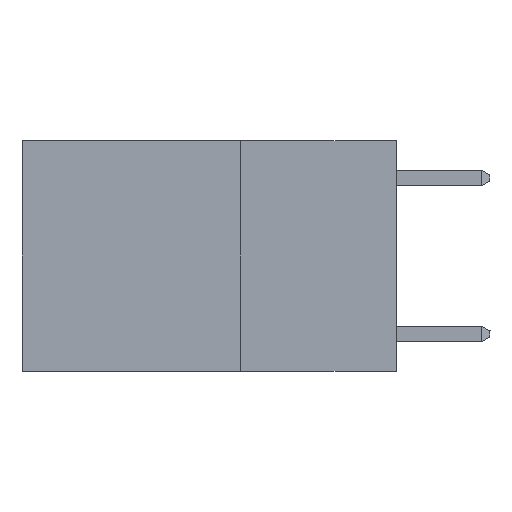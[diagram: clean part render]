
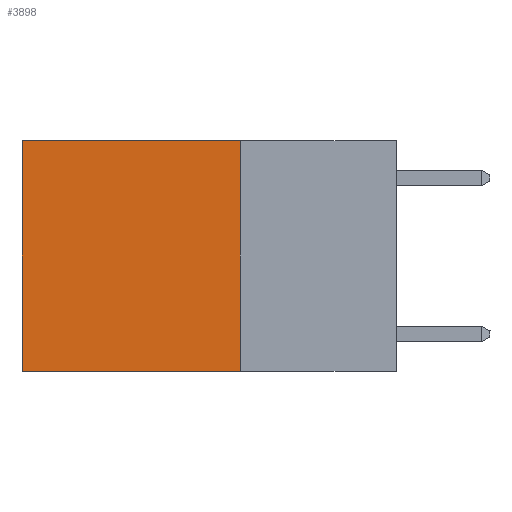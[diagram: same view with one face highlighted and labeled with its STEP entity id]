
A CAD part, left-side view. The second image highlights one B-rep face of the part: STEP entity #3898.
In plain terms, the highlighted planar face has unit normal (-1, 0, 0).
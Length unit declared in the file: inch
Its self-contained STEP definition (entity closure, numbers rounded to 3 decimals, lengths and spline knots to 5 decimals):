
#273 = DIRECTION ( 'NONE',  ( 0., 1., 0. ) ) ;
#285 = VERTEX_POINT ( 'NONE', #8281 ) ;
#292 = VECTOR ( 'NONE', #5040, 39.37008 ) ;
#549 = ORIENTED_EDGE ( 'NONE', *, *, #10072, .T. ) ;
#563 = ORIENTED_EDGE ( 'NONE', *, *, #4744, .F. ) ;
#580 = ORIENTED_EDGE ( 'NONE', *, *, #9404, .F. ) ;
#590 = ORIENTED_EDGE ( 'NONE', *, *, #4892, .T. ) ;
#812 = LINE ( 'NONE', #6621, #292 ) ;
#884 = CARTESIAN_POINT ( 'NONE',  ( 0.2625, 0.6, -0.37 ) ) ;
#2887 = VERTEX_POINT ( 'NONE', #884 ) ;
#3314 = VECTOR ( 'NONE', #273, 39.37008 ) ;
#3546 = CARTESIAN_POINT ( 'NONE',  ( 0.2625, 0.25, -0.37 ) ) ;
#3734 = AXIS2_PLACEMENT_3D ( 'NONE', #4271, #4194, #4180 ) ;
#3898 = ADVANCED_FACE ( 'NONE', ( #6685 ), #4234, .F. ) ;
#4180 = DIRECTION ( 'NONE',  ( 0., 0., -1. ) ) ;
#4194 = DIRECTION ( 'NONE',  ( 1., 0., 0. ) ) ;
#4210 = VERTEX_POINT ( 'NONE', #8242 ) ;
#4234 = PLANE ( 'NONE',  #3734 ) ;
#4271 = CARTESIAN_POINT ( 'NONE',  ( 0.2625, 0.25, 0. ) ) ;
#4431 = DIRECTION ( 'NONE',  ( 0., 0., -1. ) ) ;
#4452 = LINE ( 'NONE', #3546, #6771 ) ;
#4456 = DIRECTION ( 'NONE',  ( 0., 1., 0. ) ) ;
#4744 = EDGE_CURVE ( 'NONE', #285, #2887, #4452, .T. ) ;
#4892 = EDGE_CURVE ( 'NONE', #4210, #6890, #9446, .T. ) ;
#5040 = DIRECTION ( 'NONE',  ( 0., 0., -1. ) ) ;
#6621 = CARTESIAN_POINT ( 'NONE',  ( 0.2625, 0.6, 0. ) ) ;
#6685 = FACE_OUTER_BOUND ( 'NONE', #7329, .T. ) ;
#6771 = VECTOR ( 'NONE', #4456, 39.37008 ) ;
#6864 = CARTESIAN_POINT ( 'NONE',  ( 0.2625, 0.25, 0. ) ) ;
#6890 = VERTEX_POINT ( 'NONE', #7118 ) ;
#7043 = VECTOR ( 'NONE', #4431, 39.37008 ) ;
#7118 = CARTESIAN_POINT ( 'NONE',  ( 0.2625, 0.6, 0. ) ) ;
#7329 = EDGE_LOOP ( 'NONE', ( #549, #563, #580, #590 ) ) ;
#8242 = CARTESIAN_POINT ( 'NONE',  ( 0.2625, 0.25, 0. ) ) ;
#8281 = CARTESIAN_POINT ( 'NONE',  ( 0.2625, 0.25, -0.37 ) ) ;
#8492 = LINE ( 'NONE', #8920, #7043 ) ;
#8920 = CARTESIAN_POINT ( 'NONE',  ( 0.2625, 0.25, 0. ) ) ;
#9404 = EDGE_CURVE ( 'NONE', #4210, #285, #8492, .T. ) ;
#9446 = LINE ( 'NONE', #6864, #3314 ) ;
#10072 = EDGE_CURVE ( 'NONE', #6890, #2887, #812, .T. ) ;
